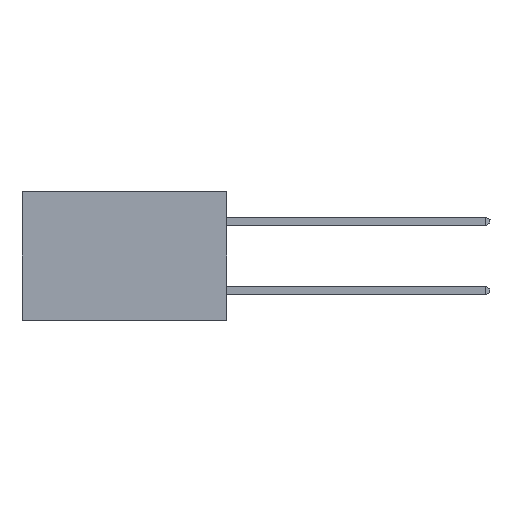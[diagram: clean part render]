
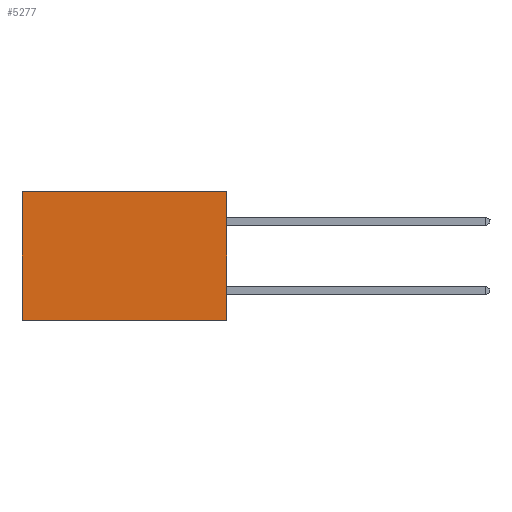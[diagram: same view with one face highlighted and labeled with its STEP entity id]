
A CAD part, left-side view. The second image highlights one B-rep face of the part: STEP entity #5277.
In plain terms, the highlighted planar face has unit normal (-1, 0, 0).
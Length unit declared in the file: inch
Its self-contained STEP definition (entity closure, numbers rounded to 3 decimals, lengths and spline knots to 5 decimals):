
#324 = LINE ( 'NONE', #5931, #8667 ) ;
#666 = CARTESIAN_POINT ( 'NONE',  ( 0.277, 0.59, 0. ) ) ;
#688 = DIRECTION ( 'NONE',  ( 0., 0., -1. ) ) ;
#1075 = CARTESIAN_POINT ( 'NONE',  ( 0.277, 0.59, -0.37 ) ) ;
#1488 = DIRECTION ( 'NONE',  ( 0., 0., -1. ) ) ;
#1564 = VERTEX_POINT ( 'NONE', #666 ) ;
#1750 = DIRECTION ( 'NONE',  ( 1., 0., 0. ) ) ;
#1881 = PLANE ( 'NONE',  #2284 ) ;
#1960 = LINE ( 'NONE', #6578, #9749 ) ;
#2032 = EDGE_CURVE ( 'NONE', #9711, #2383, #1960, .T. ) ;
#2206 = EDGE_CURVE ( 'NONE', #1564, #2383, #324, .T. ) ;
#2284 = AXIS2_PLACEMENT_3D ( 'NONE', #2518, #1750, #1488 ) ;
#2383 = VERTEX_POINT ( 'NONE', #1075 ) ;
#2518 = CARTESIAN_POINT ( 'NONE',  ( 0.277, 0., -0.37 ) ) ;
#2552 = LINE ( 'NONE', #4893, #8174 ) ;
#3292 = EDGE_CURVE ( 'NONE', #3666, #1564, #4987, .T. ) ;
#3363 = EDGE_CURVE ( 'NONE', #3666, #9711, #2552, .T. ) ;
#3666 = VERTEX_POINT ( 'NONE', #5229 ) ;
#3800 = ORIENTED_EDGE ( 'NONE', *, *, #2032, .F. ) ;
#4713 = VECTOR ( 'NONE', #6771, 39.37008 ) ;
#4844 = DIRECTION ( 'NONE',  ( 0., 0., -1. ) ) ;
#4893 = CARTESIAN_POINT ( 'NONE',  ( 0.277, 0., -0.37 ) ) ;
#4987 = LINE ( 'NONE', #6803, #4713 ) ;
#5229 = CARTESIAN_POINT ( 'NONE',  ( 0.277, 0., 0. ) ) ;
#5277 = ADVANCED_FACE ( 'NONE', ( #7902 ), #1881, .F. ) ;
#5645 = EDGE_LOOP ( 'NONE', ( #6625, #3800, #8715, #8869 ) ) ;
#5931 = CARTESIAN_POINT ( 'NONE',  ( 0.277, 0.59, -0.37 ) ) ;
#6381 = CARTESIAN_POINT ( 'NONE',  ( 0.277, 0., -0.37 ) ) ;
#6578 = CARTESIAN_POINT ( 'NONE',  ( 0.277, 0., -0.37 ) ) ;
#6625 = ORIENTED_EDGE ( 'NONE', *, *, #2206, .T. ) ;
#6771 = DIRECTION ( 'NONE',  ( 0., 1., 0. ) ) ;
#6803 = CARTESIAN_POINT ( 'NONE',  ( 0.277, 0., 0. ) ) ;
#7559 = DIRECTION ( 'NONE',  ( 0., 1., 0. ) ) ;
#7902 = FACE_OUTER_BOUND ( 'NONE', #5645, .T. ) ;
#8174 = VECTOR ( 'NONE', #4844, 39.37008 ) ;
#8667 = VECTOR ( 'NONE', #688, 39.37008 ) ;
#8715 = ORIENTED_EDGE ( 'NONE', *, *, #3363, .F. ) ;
#8869 = ORIENTED_EDGE ( 'NONE', *, *, #3292, .T. ) ;
#9711 = VERTEX_POINT ( 'NONE', #6381 ) ;
#9749 = VECTOR ( 'NONE', #7559, 39.37008 ) ;
